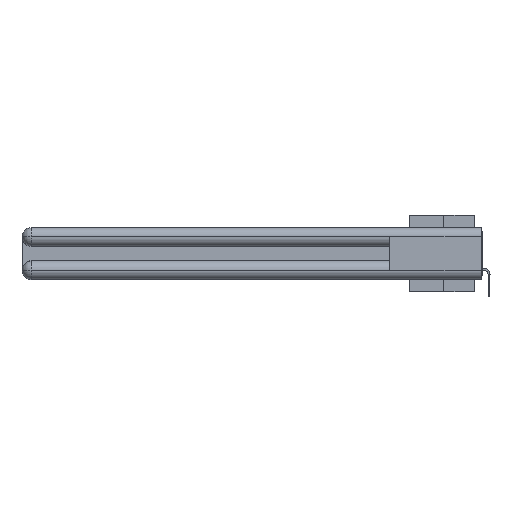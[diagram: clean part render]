
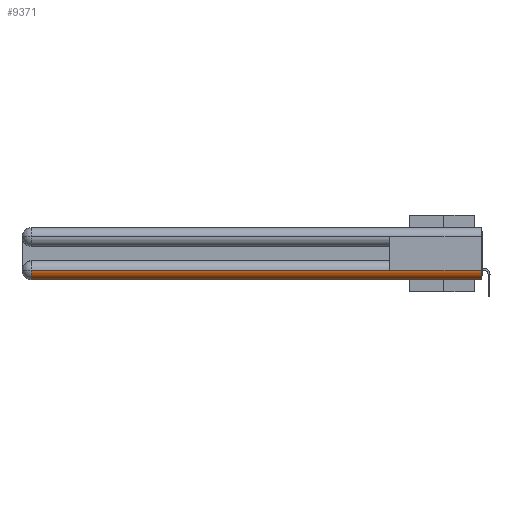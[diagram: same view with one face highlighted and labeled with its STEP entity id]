
A CAD part, left-side view. The second image highlights one B-rep face of the part: STEP entity #9371.
In plain terms, the highlighted cylindrical face has radius 1.562 mm (diameter 3.124 mm), a partial arc.
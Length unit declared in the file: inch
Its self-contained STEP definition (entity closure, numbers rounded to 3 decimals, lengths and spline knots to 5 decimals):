
#141 = VERTEX_POINT ( 'NONE', #18235 ) ;
#880 = CARTESIAN_POINT ( 'NONE',  ( 0.0615, 0., -0.2785 ) ) ;
#2252 = CIRCLE ( 'NONE', #2287, 0.0615 ) ;
#2287 = AXIS2_PLACEMENT_3D ( 'NONE', #21788, #37445, #6512 ) ;
#2819 = DIRECTION ( 'NONE',  ( 0., -1., 0. ) ) ;
#5721 = CARTESIAN_POINT ( 'NONE',  ( 0., 0., -0.2785 ) ) ;
#6098 = ORIENTED_EDGE ( 'NONE', *, *, #15456, .F. ) ;
#6512 = DIRECTION ( 'NONE',  ( 0., 0., 1. ) ) ;
#6876 = CARTESIAN_POINT ( 'NONE',  ( 0.0615, 0., -0.34 ) ) ;
#6997 = DIRECTION ( 'NONE',  ( 0., 0., -1. ) ) ;
#8396 = CIRCLE ( 'NONE', #37646, 0.0615 ) ;
#9371 = ADVANCED_FACE ( 'NONE', ( #28777 ), #22468, .T. ) ;
#10058 = EDGE_CURVE ( 'NONE', #12946, #15024, #26015, .T. ) ;
#10591 = LINE ( 'NONE', #32775, #37622 ) ;
#11764 = CARTESIAN_POINT ( 'NONE',  ( 0., 0.6, -0.2785 ) ) ;
#12946 = VERTEX_POINT ( 'NONE', #37797 ) ;
#14627 = AXIS2_PLACEMENT_3D ( 'NONE', #880, #34880, #6997 ) ;
#15024 = VERTEX_POINT ( 'NONE', #31371 ) ;
#15406 = DIRECTION ( 'NONE',  ( 0., 1., 0. ) ) ;
#15456 = EDGE_CURVE ( 'NONE', #16180, #12946, #8396, .T. ) ;
#16180 = VERTEX_POINT ( 'NONE', #5721 ) ;
#16498 = EDGE_CURVE ( 'NONE', #31262, #16180, #10591, .T. ) ;
#18235 = CARTESIAN_POINT ( 'NONE',  ( 0., 2.94, -0.2785 ) ) ;
#20570 = DIRECTION ( 'NONE',  ( 0., -1., 0. ) ) ;
#21788 = CARTESIAN_POINT ( 'NONE',  ( 0.0615, 2.94, -0.2785 ) ) ;
#22371 = ORIENTED_EDGE ( 'NONE', *, *, #36955, .T. ) ;
#22468 = CYLINDRICAL_SURFACE ( 'NONE', #14627, 0.0615 ) ;
#22469 = VECTOR ( 'NONE', #25808, 39.37008 ) ;
#24017 = CARTESIAN_POINT ( 'NONE',  ( 0.0615, 0., -0.2785 ) ) ;
#25808 = DIRECTION ( 'NONE',  ( 0., 1., 0. ) ) ;
#26015 = LINE ( 'NONE', #6876, #22469 ) ;
#27652 = DIRECTION ( 'NONE',  ( 1., 0., 0. ) ) ;
#28611 = EDGE_LOOP ( 'NONE', ( #22371, #36195, #38668, #6098, #33585 ) ) ;
#28777 = FACE_OUTER_BOUND ( 'NONE', #28611, .T. ) ;
#30482 = LINE ( 'NONE', #39840, #38489 ) ;
#31262 = VERTEX_POINT ( 'NONE', #11764 ) ;
#31371 = CARTESIAN_POINT ( 'NONE',  ( 0.0615, 2.94, -0.34 ) ) ;
#32775 = CARTESIAN_POINT ( 'NONE',  ( 0., 0., -0.2785 ) ) ;
#33585 = ORIENTED_EDGE ( 'NONE', *, *, #16498, .F. ) ;
#34880 = DIRECTION ( 'NONE',  ( 0., -1., 0. ) ) ;
#36195 = ORIENTED_EDGE ( 'NONE', *, *, #40071, .T. ) ;
#36955 = EDGE_CURVE ( 'NONE', #31262, #141, #30482, .T. ) ;
#37445 = DIRECTION ( 'NONE',  ( 0., -1., 0. ) ) ;
#37622 = VECTOR ( 'NONE', #20570, 39.37008 ) ;
#37646 = AXIS2_PLACEMENT_3D ( 'NONE', #24017, #2819, #27652 ) ;
#37797 = CARTESIAN_POINT ( 'NONE',  ( 0.0615, 0., -0.34 ) ) ;
#38489 = VECTOR ( 'NONE', #15406, 39.37008 ) ;
#38668 = ORIENTED_EDGE ( 'NONE', *, *, #10058, .F. ) ;
#39840 = CARTESIAN_POINT ( 'NONE',  ( 0., 0., -0.2785 ) ) ;
#40071 = EDGE_CURVE ( 'NONE', #141, #15024, #2252, .T. ) ;
